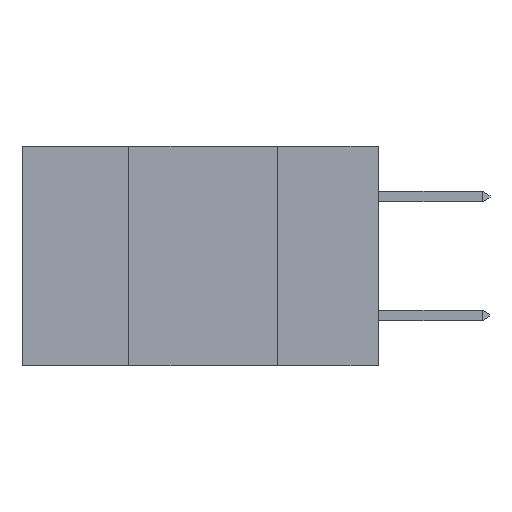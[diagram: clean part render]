
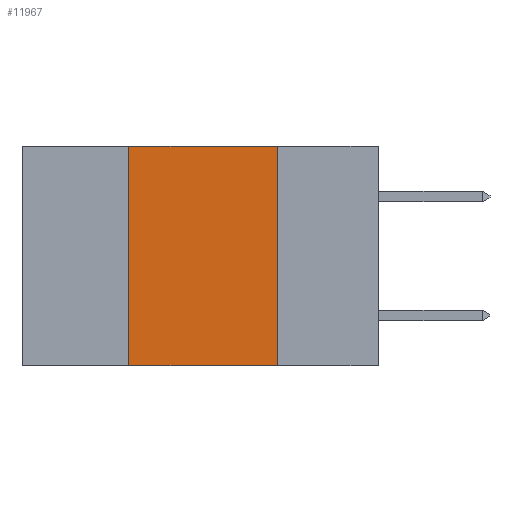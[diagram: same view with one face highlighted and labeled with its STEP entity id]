
A CAD part, left-side view. The second image highlights one B-rep face of the part: STEP entity #11967.
In plain terms, the highlighted planar face has unit normal (-1, 0, 0).
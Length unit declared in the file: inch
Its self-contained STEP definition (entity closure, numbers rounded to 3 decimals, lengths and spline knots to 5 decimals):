
#9 = CARTESIAN_POINT ( 'NONE',  ( 0., 0.6, 0. ) ) ;
#186 = CARTESIAN_POINT ( 'NONE',  ( 0., 0.6, -0.37 ) ) ;
#245 = VERTEX_POINT ( 'NONE', #8827 ) ;
#1019 = CARTESIAN_POINT ( 'NONE',  ( 0., 0.42, 0. ) ) ;
#1076 = LINE ( 'NONE', #11381, #10259 ) ;
#1108 = FACE_OUTER_BOUND ( 'NONE', #10178, .T. ) ;
#1146 = DIRECTION ( 'NONE',  ( 0., 0., -1. ) ) ;
#1612 = VECTOR ( 'NONE', #10637, 39.37008 ) ;
#1883 = ORIENTED_EDGE ( 'NONE', *, *, #12140, .F. ) ;
#2301 = ORIENTED_EDGE ( 'NONE', *, *, #6922, .F. ) ;
#2927 = VERTEX_POINT ( 'NONE', #1019 ) ;
#3300 = DIRECTION ( 'NONE',  ( 0., 0., 1. ) ) ;
#3353 = VERTEX_POINT ( 'NONE', #4951 ) ;
#3369 = EDGE_CURVE ( 'NONE', #245, #2927, #9272, .T. ) ;
#3765 = CARTESIAN_POINT ( 'NONE',  ( 0., 0.17, 0. ) ) ;
#4691 = CARTESIAN_POINT ( 'NONE',  ( 0., 0.17, -0.37 ) ) ;
#4746 = LINE ( 'NONE', #3765, #1612 ) ;
#4951 = CARTESIAN_POINT ( 'NONE',  ( 0., 0.17, 0. ) ) ;
#4979 = CARTESIAN_POINT ( 'NONE',  ( 0., 0.42, 0. ) ) ;
#5513 = VECTOR ( 'NONE', #3300, 39.37008 ) ;
#6837 = VECTOR ( 'NONE', #9406, 39.37008 ) ;
#6922 = EDGE_CURVE ( 'NONE', #2927, #3353, #1076, .T. ) ;
#8080 = DIRECTION ( 'NONE',  ( 1., 0., 0. ) ) ;
#8686 = EDGE_CURVE ( 'NONE', #245, #10465, #12801, .T. ) ;
#8827 = CARTESIAN_POINT ( 'NONE',  ( 0., 0.42, -0.37 ) ) ;
#9272 = LINE ( 'NONE', #4979, #5513 ) ;
#9406 = DIRECTION ( 'NONE',  ( 0., -1., 0. ) ) ;
#9435 = AXIS2_PLACEMENT_3D ( 'NONE', #9, #8080, #1146 ) ;
#9602 = ORIENTED_EDGE ( 'NONE', *, *, #8686, .T. ) ;
#10178 = EDGE_LOOP ( 'NONE', ( #1883, #2301, #11942, #9602 ) ) ;
#10259 = VECTOR ( 'NONE', #11527, 39.37008 ) ;
#10465 = VERTEX_POINT ( 'NONE', #4691 ) ;
#10637 = DIRECTION ( 'NONE',  ( 0., 0., -1. ) ) ;
#11381 = CARTESIAN_POINT ( 'NONE',  ( 0., 0.6, 0. ) ) ;
#11527 = DIRECTION ( 'NONE',  ( 0., -1., 0. ) ) ;
#11942 = ORIENTED_EDGE ( 'NONE', *, *, #3369, .F. ) ;
#11967 = ADVANCED_FACE ( 'NONE', ( #1108 ), #13610, .F. ) ;
#12140 = EDGE_CURVE ( 'NONE', #3353, #10465, #4746, .T. ) ;
#12801 = LINE ( 'NONE', #186, #6837 ) ;
#13610 = PLANE ( 'NONE',  #9435 ) ;
